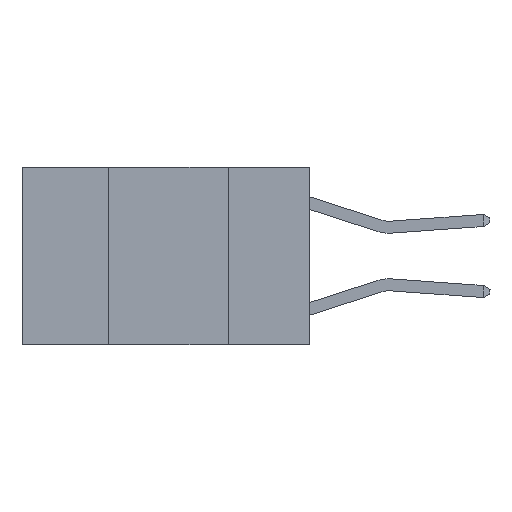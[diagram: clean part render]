
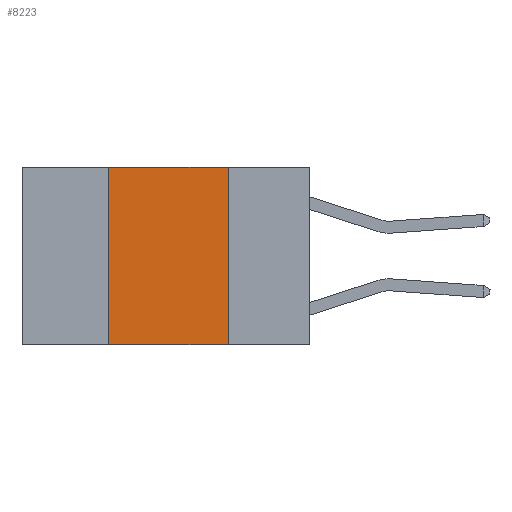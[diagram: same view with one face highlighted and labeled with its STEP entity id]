
A CAD part, left-side view. The second image highlights one B-rep face of the part: STEP entity #8223.
In plain terms, the highlighted planar face has unit normal (-1, 0, 0).
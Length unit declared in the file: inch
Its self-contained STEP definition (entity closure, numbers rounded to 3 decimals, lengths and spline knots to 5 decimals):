
#399 = DIRECTION ( 'NONE',  ( 0., 0., 1. ) ) ;
#549 = CARTESIAN_POINT ( 'NONE',  ( 0., 0.42, 0. ) ) ;
#833 = ORIENTED_EDGE ( 'NONE', *, *, #2770, .F. ) ;
#1013 = VERTEX_POINT ( 'NONE', #10044 ) ;
#1375 = VERTEX_POINT ( 'NONE', #7560 ) ;
#1521 = CARTESIAN_POINT ( 'NONE',  ( 0., 0.6, 0. ) ) ;
#1806 = CARTESIAN_POINT ( 'NONE',  ( 0., 0.6, 0. ) ) ;
#2196 = DIRECTION ( 'NONE',  ( 0., 0., -1. ) ) ;
#2770 = EDGE_CURVE ( 'NONE', #4983, #1375, #6212, .T. ) ;
#3129 = VECTOR ( 'NONE', #8695, 39.37008 ) ;
#3643 = VERTEX_POINT ( 'NONE', #8101 ) ;
#4173 = AXIS2_PLACEMENT_3D ( 'NONE', #1806, #6605, #5880 ) ;
#4281 = FACE_OUTER_BOUND ( 'NONE', #5051, .T. ) ;
#4431 = LINE ( 'NONE', #6029, #5618 ) ;
#4947 = EDGE_CURVE ( 'NONE', #1013, #4983, #9775, .T. ) ;
#4983 = VERTEX_POINT ( 'NONE', #549 ) ;
#5051 = EDGE_LOOP ( 'NONE', ( #9864, #833, #5782, #7375 ) ) ;
#5202 = DIRECTION ( 'NONE',  ( 0., -1., 0. ) ) ;
#5618 = VECTOR ( 'NONE', #5202, 39.37008 ) ;
#5782 = ORIENTED_EDGE ( 'NONE', *, *, #4947, .F. ) ;
#5880 = DIRECTION ( 'NONE',  ( 0., 0., -1. ) ) ;
#6029 = CARTESIAN_POINT ( 'NONE',  ( 0., 0.6, -0.37 ) ) ;
#6212 = LINE ( 'NONE', #1521, #3129 ) ;
#6331 = EDGE_CURVE ( 'NONE', #1375, #3643, #7679, .T. ) ;
#6333 = EDGE_CURVE ( 'NONE', #1013, #3643, #4431, .T. ) ;
#6503 = PLANE ( 'NONE',  #4173 ) ;
#6605 = DIRECTION ( 'NONE',  ( 1., 0., 0. ) ) ;
#7375 = ORIENTED_EDGE ( 'NONE', *, *, #6333, .T. ) ;
#7560 = CARTESIAN_POINT ( 'NONE',  ( 0., 0.17, 0. ) ) ;
#7679 = LINE ( 'NONE', #9181, #9578 ) ;
#8101 = CARTESIAN_POINT ( 'NONE',  ( 0., 0.17, -0.37 ) ) ;
#8223 = ADVANCED_FACE ( 'NONE', ( #4281 ), #6503, .F. ) ;
#8327 = CARTESIAN_POINT ( 'NONE',  ( 0., 0.42, 0. ) ) ;
#8660 = VECTOR ( 'NONE', #399, 39.37008 ) ;
#8695 = DIRECTION ( 'NONE',  ( 0., -1., 0. ) ) ;
#9181 = CARTESIAN_POINT ( 'NONE',  ( 0., 0.17, 0. ) ) ;
#9578 = VECTOR ( 'NONE', #2196, 39.37008 ) ;
#9775 = LINE ( 'NONE', #8327, #8660 ) ;
#9864 = ORIENTED_EDGE ( 'NONE', *, *, #6331, .F. ) ;
#10044 = CARTESIAN_POINT ( 'NONE',  ( 0., 0.42, -0.37 ) ) ;
